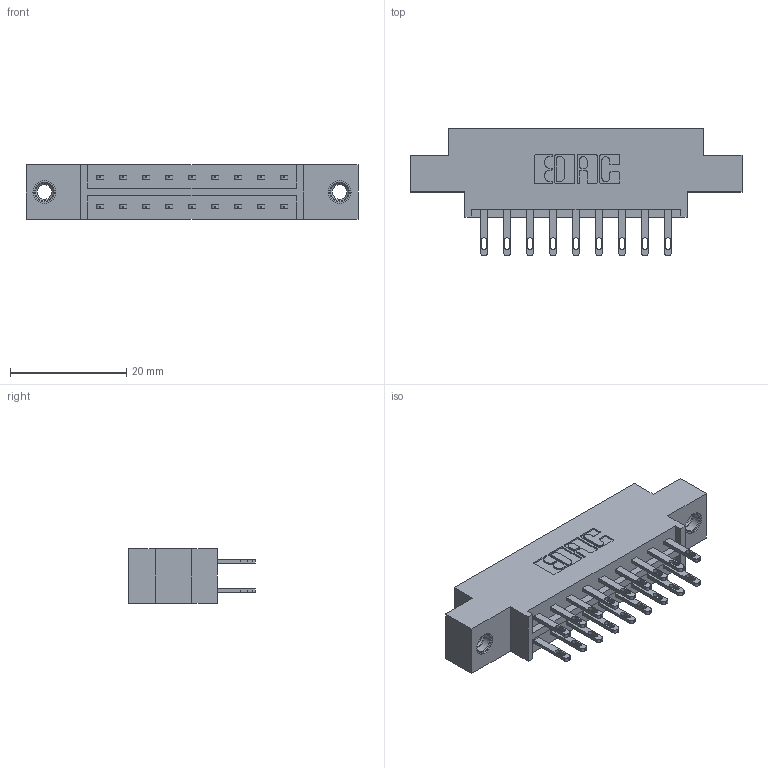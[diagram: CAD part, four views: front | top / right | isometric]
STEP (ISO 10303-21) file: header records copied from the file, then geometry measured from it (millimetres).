
FILE_DESCRIPTION (( 'STEP AP203' ), '1' );
FILE_NAME ('833-018-500-807.STEP', '2020-05-31T20:55:30', ( '' ), ( '' ), 'SwSTEP 2.0', 'SolidWorks 2020', '' );
FILE_SCHEMA (( 'CONFIG_CONTROL_DESIGN' ));
Length unit declared in the file: inch
Products named in the file (4): 345-250-001_345-250-005-103; 345-292-001_345-293-100; 833 Part_Offset - .156 Dia - TI; 833-018-500-807
Assembly tree (21 placements, depth 2):
  833-018-500-807
    833 Part_Offset - .156 Dia - TI
    345-292-001_345-293-100  x18
    345-250-001_345-250-005-103  x2
Bounding box: 57.2 x 21.85 x 9.4 mm (x, y, z)
Volume: 5345 mm3; surface area: 6417.5 mm2
Topology: 21 solids, 21 shells, 1042 faces, 3105 edges, 2062 vertices
Faces by surface type: plane 646, cylinder 380, cone 12, torus 4
Entity records: 11306 total; most frequent: CARTESIAN_POINT 1897, ORIENTED_EDGE 1826, DIRECTION 1711, EDGE_CURVE 913, LINE 761, VECTOR 761, VERTEX_POINT 604, AXIS2_PLACEMENT_3D 475
